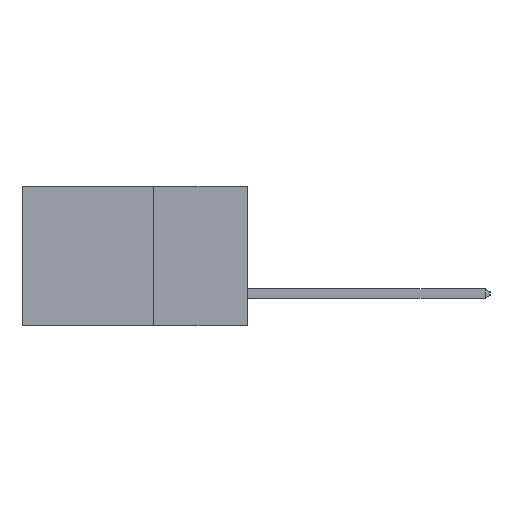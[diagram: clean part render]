
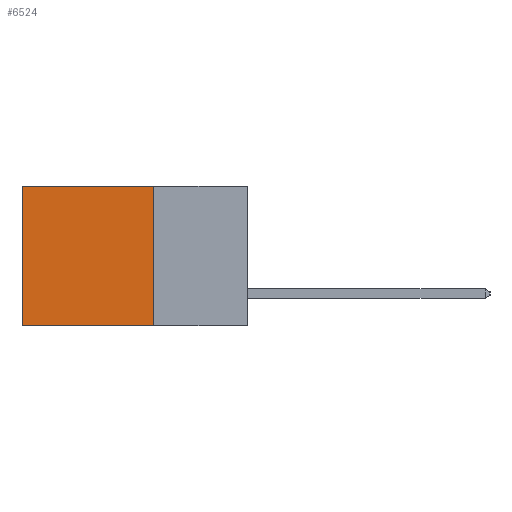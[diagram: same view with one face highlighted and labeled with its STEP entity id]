
A CAD part, left-side view. The second image highlights one B-rep face of the part: STEP entity #6524.
In plain terms, the highlighted planar face has unit normal (-1, 0, 0).
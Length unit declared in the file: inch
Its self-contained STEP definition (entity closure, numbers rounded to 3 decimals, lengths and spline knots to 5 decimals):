
#1499 = VERTEX_POINT ( 'NONE', #2052 ) ;
#1846 = CARTESIAN_POINT ( 'NONE',  ( 0.2615, 0.6, -0.37 ) ) ;
#1962 = EDGE_CURVE ( 'NONE', #1499, #11090, #11557, .T. ) ;
#1970 = ORIENTED_EDGE ( 'NONE', *, *, #8851, .T. ) ;
#2049 = VECTOR ( 'NONE', #5051, 39.37008 ) ;
#2052 = CARTESIAN_POINT ( 'NONE',  ( 0.2615, 0.25, 0. ) ) ;
#2189 = VERTEX_POINT ( 'NONE', #12289 ) ;
#2842 = CARTESIAN_POINT ( 'NONE',  ( 0.2615, 0.25, -0.37 ) ) ;
#4084 = VECTOR ( 'NONE', #4454, 39.37008 ) ;
#4333 = ORIENTED_EDGE ( 'NONE', *, *, #16771, .F. ) ;
#4454 = DIRECTION ( 'NONE',  ( 0., 1., 0. ) ) ;
#5051 = DIRECTION ( 'NONE',  ( 0., 0., -1. ) ) ;
#5266 = VECTOR ( 'NONE', #10597, 39.37008 ) ;
#6239 = CARTESIAN_POINT ( 'NONE',  ( 0.2615, 0.25, 0. ) ) ;
#6524 = ADVANCED_FACE ( 'NONE', ( #12598 ), #6937, .F. ) ;
#6904 = DIRECTION ( 'NONE',  ( 0., 0., -1. ) ) ;
#6937 = PLANE ( 'NONE',  #14158 ) ;
#7004 = DIRECTION ( 'NONE',  ( 0., 0., -1. ) ) ;
#7971 = ORIENTED_EDGE ( 'NONE', *, *, #1962, .T. ) ;
#8851 = EDGE_CURVE ( 'NONE', #11090, #17003, #10420, .T. ) ;
#10420 = LINE ( 'NONE', #15605, #2049 ) ;
#10559 = VECTOR ( 'NONE', #6904, 39.37008 ) ;
#10597 = DIRECTION ( 'NONE',  ( 0., 1., 0. ) ) ;
#11090 = VERTEX_POINT ( 'NONE', #16330 ) ;
#11557 = LINE ( 'NONE', #6239, #5266 ) ;
#12277 = EDGE_LOOP ( 'NONE', ( #1970, #4333, #18671, #7971 ) ) ;
#12289 = CARTESIAN_POINT ( 'NONE',  ( 0.2615, 0.25, -0.37 ) ) ;
#12598 = FACE_OUTER_BOUND ( 'NONE', #12277, .T. ) ;
#14158 = AXIS2_PLACEMENT_3D ( 'NONE', #14525, #15951, #7004 ) ;
#14181 = EDGE_CURVE ( 'NONE', #1499, #2189, #14476, .T. ) ;
#14428 = CARTESIAN_POINT ( 'NONE',  ( 0.2615, 0.25, -0.37 ) ) ;
#14476 = LINE ( 'NONE', #14428, #10559 ) ;
#14525 = CARTESIAN_POINT ( 'NONE',  ( 0.2615, 0.25, -0.37 ) ) ;
#15605 = CARTESIAN_POINT ( 'NONE',  ( 0.2615, 0.6, -0.37 ) ) ;
#15951 = DIRECTION ( 'NONE',  ( 1., 0., 0. ) ) ;
#16137 = LINE ( 'NONE', #2842, #4084 ) ;
#16330 = CARTESIAN_POINT ( 'NONE',  ( 0.2615, 0.6, 0. ) ) ;
#16771 = EDGE_CURVE ( 'NONE', #2189, #17003, #16137, .T. ) ;
#17003 = VERTEX_POINT ( 'NONE', #1846 ) ;
#18671 = ORIENTED_EDGE ( 'NONE', *, *, #14181, .F. ) ;
